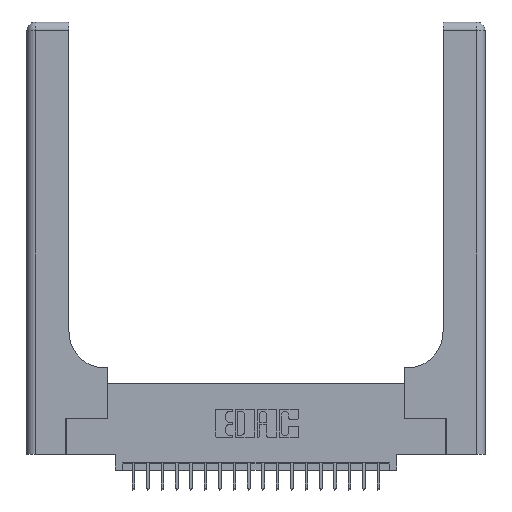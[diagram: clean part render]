
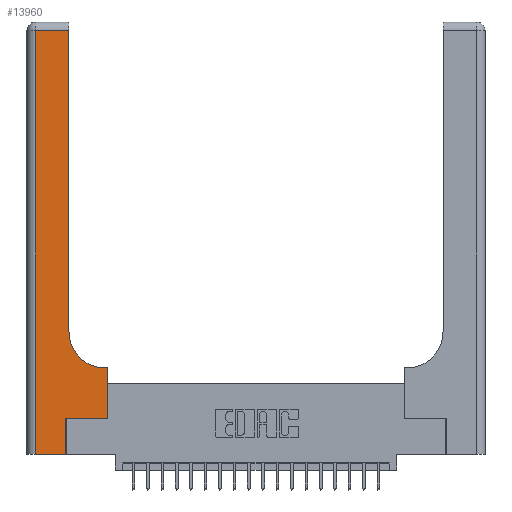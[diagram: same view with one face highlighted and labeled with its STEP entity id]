
A CAD part, top view. The second image highlights one B-rep face of the part: STEP entity #13960.
In plain terms, the highlighted planar face has unit normal (0, 0, 1).
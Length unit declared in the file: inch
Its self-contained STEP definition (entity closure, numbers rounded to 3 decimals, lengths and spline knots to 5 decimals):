
#72 = DIRECTION ( 'NONE',  ( 0., 1., 0. ) ) ;
#210 = VERTEX_POINT ( 'NONE', #18649 ) ;
#821 = CARTESIAN_POINT ( 'NONE',  ( 0.269, 0., 0.37 ) ) ;
#897 = CARTESIAN_POINT ( 'NONE',  ( 0.269, 0., 0.37 ) ) ;
#961 = DIRECTION ( 'NONE',  ( 1., 0., 0. ) ) ;
#1446 = CARTESIAN_POINT ( 'NONE',  ( 0.5585, 0.25, 0.37 ) ) ;
#2116 = EDGE_CURVE ( 'NONE', #12184, #8827, #19538, .T. ) ;
#2191 = EDGE_CURVE ( 'NONE', #210, #12184, #12013, .T. ) ;
#2450 = EDGE_CURVE ( 'NONE', #8827, #19434, #19387, .T. ) ;
#2717 = EDGE_CURVE ( 'NONE', #17327, #16901, #11399, .T. ) ;
#2776 = ORIENTED_EDGE ( 'NONE', *, *, #16377, .T. ) ;
#3416 = CARTESIAN_POINT ( 'NONE',  ( 0.2915, 0.85, 0.37 ) ) ;
#3556 = AXIS2_PLACEMENT_3D ( 'NONE', #5632, #12669, #20367 ) ;
#3923 = VECTOR ( 'NONE', #21217, 39.37008 ) ;
#3950 = LINE ( 'NONE', #12371, #14314 ) ;
#4651 = LINE ( 'NONE', #16762, #20571 ) ;
#4667 = CARTESIAN_POINT ( 'NONE',  ( 0.06, 2.94, 0.37 ) ) ;
#5632 = CARTESIAN_POINT ( 'NONE',  ( 0., 3., 0.37 ) ) ;
#5641 = EDGE_CURVE ( 'NONE', #16607, #22131, #17263, .T. ) ;
#6513 = ORIENTED_EDGE ( 'NONE', *, *, #18545, .T. ) ;
#7335 = CARTESIAN_POINT ( 'NONE',  ( 0.5585, 0.6, 0.37 ) ) ;
#7390 = CARTESIAN_POINT ( 'NONE',  ( 0., 2.94, 0.37 ) ) ;
#7593 = CARTESIAN_POINT ( 'NONE',  ( 0.2915, 2.94, 0.37 ) ) ;
#7636 = VERTEX_POINT ( 'NONE', #10827 ) ;
#7692 = EDGE_LOOP ( 'NONE', ( #8430, #10872, #17894, #2776, #10891, #6513, #16495, #11098, #15846 ) ) ;
#7863 = DIRECTION ( 'NONE',  ( 0., 0., -1. ) ) ;
#7903 = DIRECTION ( 'NONE',  ( -1., 0., 0. ) ) ;
#7944 = DIRECTION ( 'NONE',  ( 0., 1., 0. ) ) ;
#8430 = ORIENTED_EDGE ( 'NONE', *, *, #2116, .T. ) ;
#8827 = VERTEX_POINT ( 'NONE', #7593 ) ;
#9369 = CARTESIAN_POINT ( 'NONE',  ( 0.2915, 3., 0.37 ) ) ;
#9447 = AXIS2_PLACEMENT_3D ( 'NONE', #9933, #7863, #9605 ) ;
#9605 = DIRECTION ( 'NONE',  ( 1., 0., 0. ) ) ;
#9933 = CARTESIAN_POINT ( 'NONE',  ( 0.5415, 0.85, 0.37 ) ) ;
#10817 = PLANE ( 'NONE',  #3556 ) ;
#10827 = CARTESIAN_POINT ( 'NONE',  ( 0.06, 0., 0.37 ) ) ;
#10872 = ORIENTED_EDGE ( 'NONE', *, *, #2450, .T. ) ;
#10891 = ORIENTED_EDGE ( 'NONE', *, *, #2717, .T. ) ;
#10930 = VECTOR ( 'NONE', #7944, 39.37008 ) ;
#11098 = ORIENTED_EDGE ( 'NONE', *, *, #14319, .T. ) ;
#11399 = LINE ( 'NONE', #897, #10930 ) ;
#12013 = CIRCLE ( 'NONE', #9447, 0.25 ) ;
#12184 = VERTEX_POINT ( 'NONE', #3416 ) ;
#12371 = CARTESIAN_POINT ( 'NONE',  ( 0.269, 0.25, 0.37 ) ) ;
#12557 = FACE_OUTER_BOUND ( 'NONE', #7692, .T. ) ;
#12669 = DIRECTION ( 'NONE',  ( 0., 0., -1. ) ) ;
#12932 = EDGE_CURVE ( 'NONE', #19434, #7636, #19034, .T. ) ;
#13701 = CARTESIAN_POINT ( 'NONE',  ( 0.269, 0.25, 0.37 ) ) ;
#13840 = VECTOR ( 'NONE', #15461, 39.37008 ) ;
#13960 = ADVANCED_FACE ( 'NONE', ( #12557 ), #10817, .F. ) ;
#14238 = VECTOR ( 'NONE', #7903, 39.37008 ) ;
#14314 = VECTOR ( 'NONE', #14437, 39.37008 ) ;
#14319 = EDGE_CURVE ( 'NONE', #22131, #210, #21716, .T. ) ;
#14437 = DIRECTION ( 'NONE',  ( 1., 0., 0. ) ) ;
#15332 = VECTOR ( 'NONE', #18098, 39.37008 ) ;
#15461 = DIRECTION ( 'NONE',  ( 0., -1., 0. ) ) ;
#15846 = ORIENTED_EDGE ( 'NONE', *, *, #2191, .T. ) ;
#16125 = VECTOR ( 'NONE', #72, 39.37008 ) ;
#16377 = EDGE_CURVE ( 'NONE', #7636, #17327, #4651, .T. ) ;
#16495 = ORIENTED_EDGE ( 'NONE', *, *, #5641, .T. ) ;
#16607 = VERTEX_POINT ( 'NONE', #19876 ) ;
#16762 = CARTESIAN_POINT ( 'NONE',  ( 0., 0., 0.37 ) ) ;
#16901 = VERTEX_POINT ( 'NONE', #13701 ) ;
#17263 = LINE ( 'NONE', #1446, #16125 ) ;
#17327 = VERTEX_POINT ( 'NONE', #821 ) ;
#17894 = ORIENTED_EDGE ( 'NONE', *, *, #12932, .T. ) ;
#18098 = DIRECTION ( 'NONE',  ( -1., 0., 0. ) ) ;
#18545 = EDGE_CURVE ( 'NONE', #16901, #16607, #3950, .T. ) ;
#18649 = CARTESIAN_POINT ( 'NONE',  ( 0.5415, 0.6, 0.37 ) ) ;
#18918 = CARTESIAN_POINT ( 'NONE',  ( 0.06, 3., 0.37 ) ) ;
#19034 = LINE ( 'NONE', #18918, #13840 ) ;
#19387 = LINE ( 'NONE', #7390, #15332 ) ;
#19434 = VERTEX_POINT ( 'NONE', #4667 ) ;
#19538 = LINE ( 'NONE', #9369, #3923 ) ;
#19876 = CARTESIAN_POINT ( 'NONE',  ( 0.5585, 0.25, 0.37 ) ) ;
#20367 = DIRECTION ( 'NONE',  ( -1., 0., 0. ) ) ;
#20571 = VECTOR ( 'NONE', #961, 39.37008 ) ;
#21217 = DIRECTION ( 'NONE',  ( 0., 1., 0. ) ) ;
#21716 = LINE ( 'NONE', #22154, #14238 ) ;
#22131 = VERTEX_POINT ( 'NONE', #7335 ) ;
#22154 = CARTESIAN_POINT ( 'NONE',  ( 0.2915, 0.6, 0.37 ) ) ;
